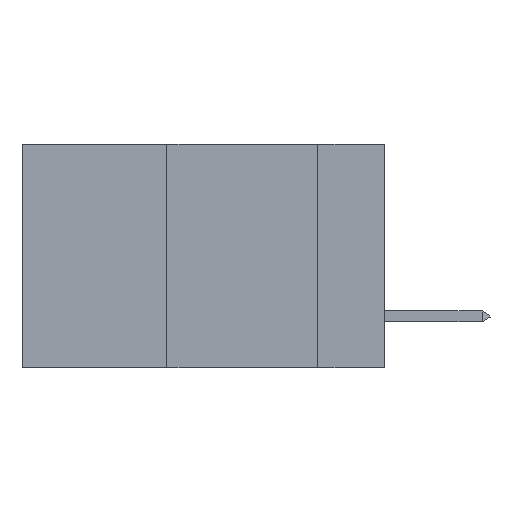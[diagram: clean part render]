
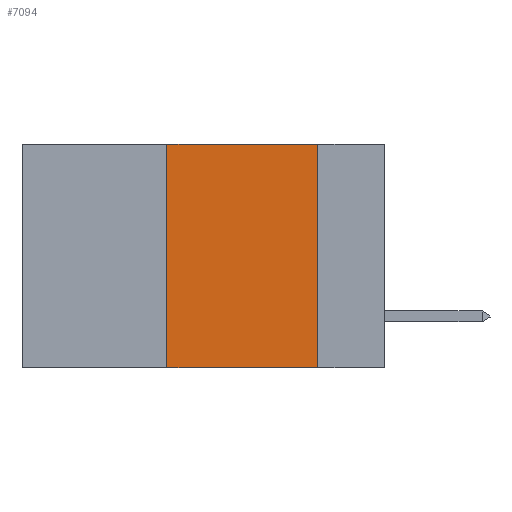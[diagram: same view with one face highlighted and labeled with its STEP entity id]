
A CAD part, left-side view. The second image highlights one B-rep face of the part: STEP entity #7094.
In plain terms, the highlighted planar face has unit normal (-1, 0, 0).
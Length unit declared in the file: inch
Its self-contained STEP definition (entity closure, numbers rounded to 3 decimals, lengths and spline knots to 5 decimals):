
#392 = VECTOR ( 'NONE', #34621, 39.37008 ) ;
#2266 = VERTEX_POINT ( 'NONE', #30477 ) ;
#3905 = CARTESIAN_POINT ( 'NONE',  ( 0., 0.6, -0.37 ) ) ;
#5039 = VECTOR ( 'NONE', #18629, 39.37008 ) ;
#5237 = VERTEX_POINT ( 'NONE', #9861 ) ;
#7094 = ADVANCED_FACE ( 'NONE', ( #44916 ), #28906, .F. ) ;
#8745 = EDGE_CURVE ( 'NONE', #13119, #5237, #13277, .T. ) ;
#8986 = ORIENTED_EDGE ( 'NONE', *, *, #8745, .F. ) ;
#9495 = LINE ( 'NONE', #3905, #34702 ) ;
#9861 = CARTESIAN_POINT ( 'NONE',  ( 0., 0.36, 0. ) ) ;
#11355 = ORIENTED_EDGE ( 'NONE', *, *, #26198, .T. ) ;
#12804 = CARTESIAN_POINT ( 'NONE',  ( 0., 0.36, 0. ) ) ;
#13119 = VERTEX_POINT ( 'NONE', #25134 ) ;
#13277 = LINE ( 'NONE', #12804, #392 ) ;
#13674 = DIRECTION ( 'NONE',  ( 0., 0., -1. ) ) ;
#13802 = DIRECTION ( 'NONE',  ( 0., -1., 0. ) ) ;
#14959 = LINE ( 'NONE', #29820, #5039 ) ;
#18629 = DIRECTION ( 'NONE',  ( 0., 0., -1. ) ) ;
#19546 = EDGE_LOOP ( 'NONE', ( #42193, #20747, #8986, #11355 ) ) ;
#20073 = EDGE_CURVE ( 'NONE', #47935, #2266, #14959, .T. ) ;
#20747 = ORIENTED_EDGE ( 'NONE', *, *, #43933, .F. ) ;
#25116 = CARTESIAN_POINT ( 'NONE',  ( 0., 0.11, 0. ) ) ;
#25134 = CARTESIAN_POINT ( 'NONE',  ( 0., 0.36, -0.37 ) ) ;
#26198 = EDGE_CURVE ( 'NONE', #13119, #2266, #9495, .T. ) ;
#28906 = PLANE ( 'NONE',  #38798 ) ;
#29820 = CARTESIAN_POINT ( 'NONE',  ( 0., 0.11, 0. ) ) ;
#30087 = DIRECTION ( 'NONE',  ( 0., -1., 0. ) ) ;
#30477 = CARTESIAN_POINT ( 'NONE',  ( 0., 0.11, -0.37 ) ) ;
#32483 = CARTESIAN_POINT ( 'NONE',  ( 0., 0.6, 0. ) ) ;
#32687 = CARTESIAN_POINT ( 'NONE',  ( 0., 0.6, 0. ) ) ;
#34621 = DIRECTION ( 'NONE',  ( 0., 0., 1. ) ) ;
#34702 = VECTOR ( 'NONE', #30087, 39.37008 ) ;
#36287 = DIRECTION ( 'NONE',  ( 1., 0., 0. ) ) ;
#38798 = AXIS2_PLACEMENT_3D ( 'NONE', #32687, #36287, #13674 ) ;
#40872 = LINE ( 'NONE', #32483, #46807 ) ;
#42193 = ORIENTED_EDGE ( 'NONE', *, *, #20073, .F. ) ;
#43933 = EDGE_CURVE ( 'NONE', #5237, #47935, #40872, .T. ) ;
#44916 = FACE_OUTER_BOUND ( 'NONE', #19546, .T. ) ;
#46807 = VECTOR ( 'NONE', #13802, 39.37008 ) ;
#47935 = VERTEX_POINT ( 'NONE', #25116 ) ;
